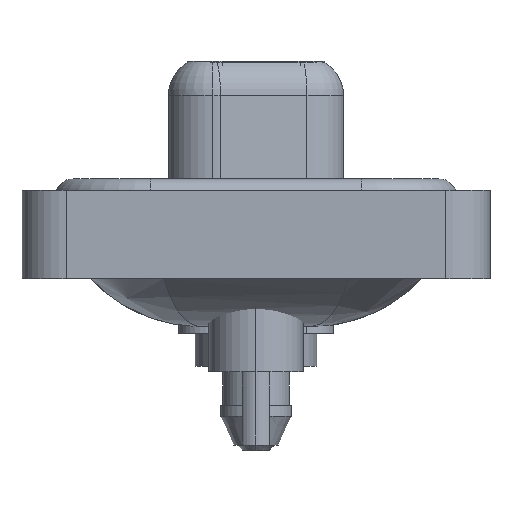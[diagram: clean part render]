
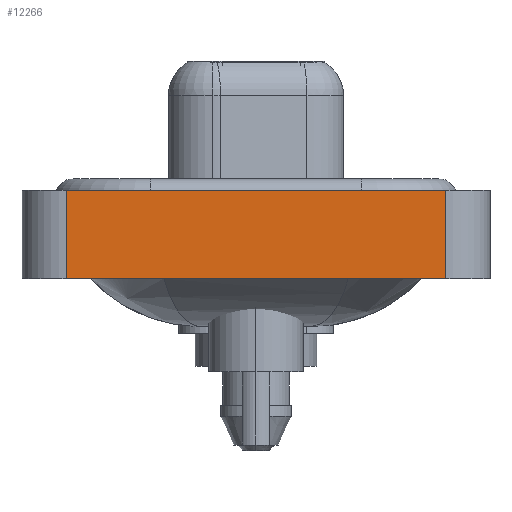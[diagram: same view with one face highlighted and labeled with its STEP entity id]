
A CAD part, left-side view. The second image highlights one B-rep face of the part: STEP entity #12266.
In plain terms, the highlighted planar face has unit normal (-1, 0, 0).
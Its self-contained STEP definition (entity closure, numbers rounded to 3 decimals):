
#710 = CARTESIAN_POINT ( 'NONE',  ( -7.3, -8.55, -3.6 ) ) ;
#1226 = LINE ( 'NONE', #6845, #8193 ) ;
#1451 = VERTEX_POINT ( 'NONE', #11361 ) ;
#1774 = ORIENTED_EDGE ( 'NONE', *, *, #16725, .T. ) ;
#2495 = EDGE_CURVE ( 'NONE', #8385, #5018, #12994, .T. ) ;
#2795 = VECTOR ( 'NONE', #8882, 1000. ) ;
#2999 = AXIS2_PLACEMENT_3D ( 'NONE', #710, #6509, #11890 ) ;
#3003 = VERTEX_POINT ( 'NONE', #7280 ) ;
#3282 = CARTESIAN_POINT ( 'NONE',  ( -7.3, 8.55, -3.6 ) ) ;
#3324 = EDGE_LOOP ( 'NONE', ( #1774, #16580, #4205, #10596 ) ) ;
#4205 = ORIENTED_EDGE ( 'NONE', *, *, #2495, .F. ) ;
#4750 = EDGE_CURVE ( 'NONE', #5018, #3003, #12110, .T. ) ;
#5018 = VERTEX_POINT ( 'NONE', #17266 ) ;
#6509 = DIRECTION ( 'NONE',  ( -1., 0., 0. ) ) ;
#6845 = CARTESIAN_POINT ( 'NONE',  ( -7.3, -8.55, -3.6 ) ) ;
#7280 = CARTESIAN_POINT ( 'NONE',  ( -7.3, -8.55, 0.4 ) ) ;
#7792 = FACE_OUTER_BOUND ( 'NONE', #3324, .T. ) ;
#7870 = EDGE_CURVE ( 'NONE', #8385, #1451, #17648, .T. ) ;
#8193 = VECTOR ( 'NONE', #9299, 1000. ) ;
#8214 = DIRECTION ( 'NONE',  ( 0., -1., 0. ) ) ;
#8385 = VERTEX_POINT ( 'NONE', #12804 ) ;
#8882 = DIRECTION ( 'NONE',  ( 0., 0., 1. ) ) ;
#9299 = DIRECTION ( 'NONE',  ( 0., 0., 1. ) ) ;
#9824 = VECTOR ( 'NONE', #8214, 1000. ) ;
#9894 = VECTOR ( 'NONE', #16595, 1000. ) ;
#10596 = ORIENTED_EDGE ( 'NONE', *, *, #7870, .T. ) ;
#10866 = CARTESIAN_POINT ( 'NONE',  ( -7.3, -8.55, -3.6 ) ) ;
#11361 = CARTESIAN_POINT ( 'NONE',  ( -7.3, -8.55, -3.6 ) ) ;
#11890 = DIRECTION ( 'NONE',  ( 0., 0., 1. ) ) ;
#12110 = LINE ( 'NONE', #17700, #9894 ) ;
#12266 = ADVANCED_FACE ( 'NONE', ( #7792 ), #16393, .T. ) ;
#12804 = CARTESIAN_POINT ( 'NONE',  ( -7.3, 8.55, -3.6 ) ) ;
#12994 = LINE ( 'NONE', #3282, #2795 ) ;
#16393 = PLANE ( 'NONE',  #2999 ) ;
#16580 = ORIENTED_EDGE ( 'NONE', *, *, #4750, .F. ) ;
#16595 = DIRECTION ( 'NONE',  ( 0., -1., 0. ) ) ;
#16725 = EDGE_CURVE ( 'NONE', #1451, #3003, #1226, .T. ) ;
#17266 = CARTESIAN_POINT ( 'NONE',  ( -7.3, 8.55, 0.4 ) ) ;
#17648 = LINE ( 'NONE', #10866, #9824 ) ;
#17700 = CARTESIAN_POINT ( 'NONE',  ( -7.3, -8.55, 0.4 ) ) ;
